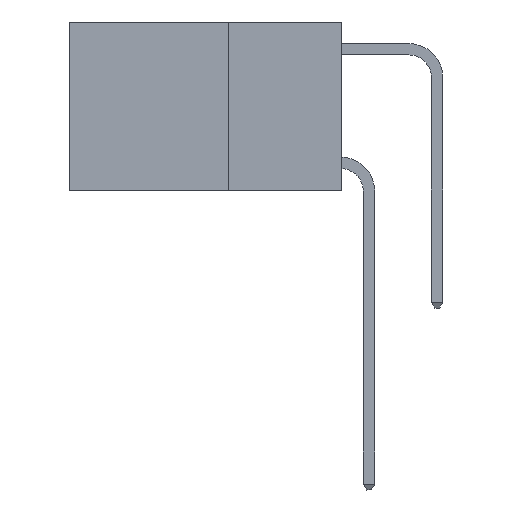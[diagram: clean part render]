
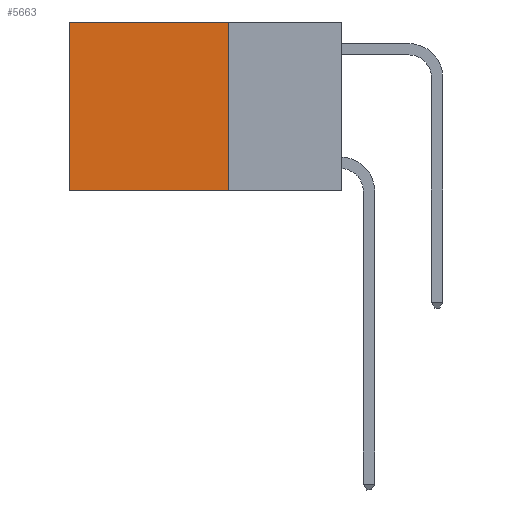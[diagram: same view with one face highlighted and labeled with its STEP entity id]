
A CAD part, left-side view. The second image highlights one B-rep face of the part: STEP entity #5663.
In plain terms, the highlighted planar face has unit normal (-1, 0, 0).
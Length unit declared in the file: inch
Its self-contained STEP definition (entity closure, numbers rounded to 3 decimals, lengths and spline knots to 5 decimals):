
#178 = CARTESIAN_POINT ( 'NONE',  ( 0.2625, 0.25, -0.37 ) ) ;
#378 = LINE ( 'NONE', #178, #4376 ) ;
#622 = DIRECTION ( 'NONE',  ( 0., 0., -1. ) ) ;
#1761 = EDGE_CURVE ( 'NONE', #4464, #3870, #10154, .T. ) ;
#2230 = CARTESIAN_POINT ( 'NONE',  ( 0.2625, 0.6, 0. ) ) ;
#2235 = VERTEX_POINT ( 'NONE', #3565 ) ;
#3416 = DIRECTION ( 'NONE',  ( 0., 0., -1. ) ) ;
#3565 = CARTESIAN_POINT ( 'NONE',  ( 0.2625, 0.6, -0.37 ) ) ;
#3870 = VERTEX_POINT ( 'NONE', #12049 ) ;
#4323 = DIRECTION ( 'NONE',  ( 1., 0., 0. ) ) ;
#4376 = VECTOR ( 'NONE', #4604, 39.37008 ) ;
#4464 = VERTEX_POINT ( 'NONE', #11085 ) ;
#4532 = CARTESIAN_POINT ( 'NONE',  ( 0.2625, 0.25, 0. ) ) ;
#4604 = DIRECTION ( 'NONE',  ( 0., 1., 0. ) ) ;
#4628 = EDGE_CURVE ( 'NONE', #13297, #2235, #11070, .T. ) ;
#4857 = CARTESIAN_POINT ( 'NONE',  ( 0.2625, 0.6, 0. ) ) ;
#4883 = CARTESIAN_POINT ( 'NONE',  ( 0.2625, 0.25, 0. ) ) ;
#5327 = ORIENTED_EDGE ( 'NONE', *, *, #5699, .F. ) ;
#5663 = ADVANCED_FACE ( 'NONE', ( #8580 ), #6430, .F. ) ;
#5699 = EDGE_CURVE ( 'NONE', #3870, #2235, #378, .T. ) ;
#5757 = DIRECTION ( 'NONE',  ( 0., 0., -1. ) ) ;
#6216 = ORIENTED_EDGE ( 'NONE', *, *, #10719, .T. ) ;
#6430 = PLANE ( 'NONE',  #10263 ) ;
#7126 = VECTOR ( 'NONE', #12236, 39.37008 ) ;
#8041 = CARTESIAN_POINT ( 'NONE',  ( 0.2625, 0.25, 0. ) ) ;
#8221 = EDGE_LOOP ( 'NONE', ( #9918, #5327, #11107, #6216 ) ) ;
#8580 = FACE_OUTER_BOUND ( 'NONE', #8221, .T. ) ;
#9918 = ORIENTED_EDGE ( 'NONE', *, *, #4628, .T. ) ;
#10154 = LINE ( 'NONE', #8041, #10313 ) ;
#10263 = AXIS2_PLACEMENT_3D ( 'NONE', #4532, #4323, #3416 ) ;
#10281 = LINE ( 'NONE', #4883, #7126 ) ;
#10313 = VECTOR ( 'NONE', #622, 39.37008 ) ;
#10719 = EDGE_CURVE ( 'NONE', #4464, #13297, #10281, .T. ) ;
#11070 = LINE ( 'NONE', #4857, #11970 ) ;
#11085 = CARTESIAN_POINT ( 'NONE',  ( 0.2625, 0.25, 0. ) ) ;
#11107 = ORIENTED_EDGE ( 'NONE', *, *, #1761, .F. ) ;
#11970 = VECTOR ( 'NONE', #5757, 39.37008 ) ;
#12049 = CARTESIAN_POINT ( 'NONE',  ( 0.2625, 0.25, -0.37 ) ) ;
#12236 = DIRECTION ( 'NONE',  ( 0., 1., 0. ) ) ;
#13297 = VERTEX_POINT ( 'NONE', #2230 ) ;
